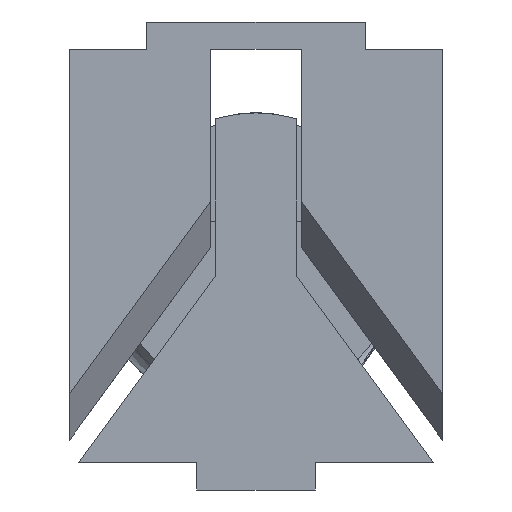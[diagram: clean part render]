
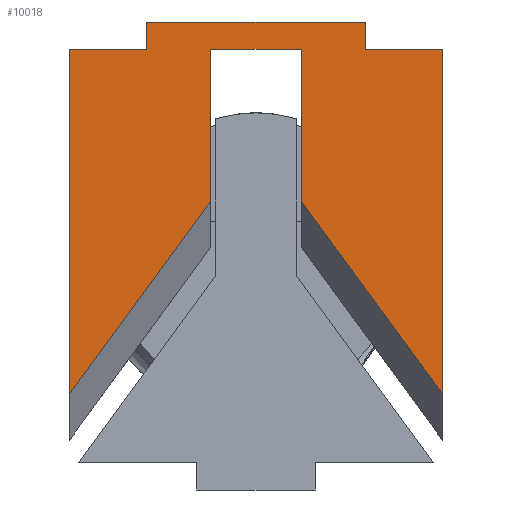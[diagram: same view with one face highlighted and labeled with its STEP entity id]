
A CAD part, front view. The second image highlights one B-rep face of the part: STEP entity #10018.
In plain terms, the highlighted planar face has unit normal (0, -1, 0).
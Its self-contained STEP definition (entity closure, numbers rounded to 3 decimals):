
#302 = VECTOR ( 'NONE', #7998, 1000. ) ;
#310 = ORIENTED_EDGE ( 'NONE', *, *, #9682, .F. ) ;
#428 = VECTOR ( 'NONE', #872, 1000. ) ;
#720 = ORIENTED_EDGE ( 'NONE', *, *, #2847, .T. ) ;
#864 = CARTESIAN_POINT ( 'NONE',  ( -12., 50., 17. ) ) ;
#872 = DIRECTION ( 'NONE',  ( 0., 0., -1. ) ) ;
#1059 = EDGE_CURVE ( 'NONE', #4661, #6381, #4968, .T. ) ;
#1181 = CARTESIAN_POINT ( 'NONE',  ( 20.5, 50., -23.919 ) ) ;
#1329 = ORIENTED_EDGE ( 'NONE', *, *, #1059, .F. ) ;
#1627 = DIRECTION ( 'NONE',  ( 0., 0., 1. ) ) ;
#1660 = CARTESIAN_POINT ( 'NONE',  ( 20.5, 50., 14. ) ) ;
#1767 = EDGE_CURVE ( 'NONE', #5907, #6381, #9399, .T. ) ;
#1841 = VECTOR ( 'NONE', #10079, 1000. ) ;
#1881 = CARTESIAN_POINT ( 'NONE',  ( -12., 50., 17. ) ) ;
#2059 = ORIENTED_EDGE ( 'NONE', *, *, #5242, .T. ) ;
#2090 = VERTEX_POINT ( 'NONE', #6871 ) ;
#2649 = CARTESIAN_POINT ( 'NONE',  ( 0., 50., 14. ) ) ;
#2847 = EDGE_CURVE ( 'NONE', #4973, #5907, #3193, .T. ) ;
#2854 = LINE ( 'NONE', #7149, #2921 ) ;
#2919 = PLANE ( 'NONE',  #5298 ) ;
#2921 = VECTOR ( 'NONE', #5198, 1000. ) ;
#3057 = CARTESIAN_POINT ( 'NONE',  ( 0.665, 50., 3.192 ) ) ;
#3060 = EDGE_CURVE ( 'NONE', #9786, #2090, #2854, .T. ) ;
#3189 = EDGE_CURVE ( 'NONE', #7574, #6319, #8959, .T. ) ;
#3193 = LINE ( 'NONE', #4187, #3800 ) ;
#3325 = CARTESIAN_POINT ( 'NONE',  ( -12., 50., 17. ) ) ;
#3366 = DIRECTION ( 'NONE',  ( 1., 0., 0. ) ) ;
#3448 = EDGE_CURVE ( 'NONE', #3493, #6377, #8599, .T. ) ;
#3468 = LINE ( 'NONE', #864, #9061 ) ;
#3493 = VERTEX_POINT ( 'NONE', #1881 ) ;
#3753 = CARTESIAN_POINT ( 'NONE',  ( -11.822, 50., -12.057 ) ) ;
#3792 = DIRECTION ( 'NONE',  ( 0., 0., 1. ) ) ;
#3800 = VECTOR ( 'NONE', #1627, 1000. ) ;
#4056 = DIRECTION ( 'NONE',  ( 0.59, 0., -0.807 ) ) ;
#4106 = CARTESIAN_POINT ( 'NONE',  ( 5., 50., -2.733 ) ) ;
#4187 = CARTESIAN_POINT ( 'NONE',  ( -5., 50., 0. ) ) ;
#4564 = VERTEX_POINT ( 'NONE', #8479 ) ;
#4588 = CARTESIAN_POINT ( 'NONE',  ( 0., 50., 14. ) ) ;
#4602 = DIRECTION ( 'NONE',  ( 0.59, 0., 0.807 ) ) ;
#4661 = VERTEX_POINT ( 'NONE', #4106 ) ;
#4705 = DIRECTION ( 'NONE',  ( 0., 0., 1. ) ) ;
#4827 = EDGE_CURVE ( 'NONE', #3493, #9786, #3468, .T. ) ;
#4846 = DIRECTION ( 'NONE',  ( 0., 0., -1. ) ) ;
#4892 = LINE ( 'NONE', #3057, #5358 ) ;
#4968 = LINE ( 'NONE', #5805, #8323 ) ;
#4973 = VERTEX_POINT ( 'NONE', #7791 ) ;
#5173 = CARTESIAN_POINT ( 'NONE',  ( -20.5, 50., 14. ) ) ;
#5198 = DIRECTION ( 'NONE',  ( 0., 0., -1. ) ) ;
#5242 = EDGE_CURVE ( 'NONE', #4564, #4973, #9868, .T. ) ;
#5298 = AXIS2_PLACEMENT_3D ( 'NONE', #8280, #6409, #4705 ) ;
#5358 = VECTOR ( 'NONE', #4056, 1000. ) ;
#5729 = CARTESIAN_POINT ( 'NONE',  ( -20.5, 50., 0. ) ) ;
#5780 = VECTOR ( 'NONE', #4846, 1000. ) ;
#5805 = CARTESIAN_POINT ( 'NONE',  ( 5., 50., 0. ) ) ;
#5907 = VERTEX_POINT ( 'NONE', #9472 ) ;
#6319 = VERTEX_POINT ( 'NONE', #1181 ) ;
#6377 = VERTEX_POINT ( 'NONE', #7035 ) ;
#6381 = VERTEX_POINT ( 'NONE', #7280 ) ;
#6409 = DIRECTION ( 'NONE',  ( 0., 1., 0. ) ) ;
#6649 = EDGE_CURVE ( 'NONE', #10498, #4564, #6877, .T. ) ;
#6693 = ORIENTED_EDGE ( 'NONE', *, *, #3060, .F. ) ;
#6871 = CARTESIAN_POINT ( 'NONE',  ( 12., 50., 14. ) ) ;
#6877 = LINE ( 'NONE', #5729, #8265 ) ;
#6915 = ORIENTED_EDGE ( 'NONE', *, *, #3189, .F. ) ;
#7035 = CARTESIAN_POINT ( 'NONE',  ( -12., 50., 14. ) ) ;
#7149 = CARTESIAN_POINT ( 'NONE',  ( 12., 50., 17. ) ) ;
#7280 = CARTESIAN_POINT ( 'NONE',  ( 5., 50., 14. ) ) ;
#7354 = ORIENTED_EDGE ( 'NONE', *, *, #3448, .T. ) ;
#7425 = CARTESIAN_POINT ( 'NONE',  ( 20.5, 50., 0. ) ) ;
#7574 = VERTEX_POINT ( 'NONE', #1660 ) ;
#7791 = CARTESIAN_POINT ( 'NONE',  ( -5., 50., -2.733 ) ) ;
#7901 = EDGE_CURVE ( 'NONE', #4661, #6319, #4892, .T. ) ;
#7962 = EDGE_CURVE ( 'NONE', #10498, #6377, #8637, .T. ) ;
#7998 = DIRECTION ( 'NONE',  ( 1., 0., 0. ) ) ;
#8187 = ORIENTED_EDGE ( 'NONE', *, *, #7901, .T. ) ;
#8228 = FACE_OUTER_BOUND ( 'NONE', #11048, .T. ) ;
#8265 = VECTOR ( 'NONE', #9255, 1000. ) ;
#8280 = CARTESIAN_POINT ( 'NONE',  ( -16., 50., -9. ) ) ;
#8323 = VECTOR ( 'NONE', #3792, 1000. ) ;
#8479 = CARTESIAN_POINT ( 'NONE',  ( -20.5, 50., -23.919 ) ) ;
#8498 = CARTESIAN_POINT ( 'NONE',  ( -12., 50., 14. ) ) ;
#8574 = VECTOR ( 'NONE', #4602, 1000. ) ;
#8599 = LINE ( 'NONE', #3325, #428 ) ;
#8637 = LINE ( 'NONE', #2649, #10555 ) ;
#8784 = ORIENTED_EDGE ( 'NONE', *, *, #6649, .T. ) ;
#8824 = ORIENTED_EDGE ( 'NONE', *, *, #1767, .T. ) ;
#8850 = LINE ( 'NONE', #4588, #302 ) ;
#8959 = LINE ( 'NONE', #7425, #5780 ) ;
#9061 = VECTOR ( 'NONE', #9541, 1000. ) ;
#9165 = ORIENTED_EDGE ( 'NONE', *, *, #4827, .F. ) ;
#9255 = DIRECTION ( 'NONE',  ( 0., 0., -1. ) ) ;
#9281 = ORIENTED_EDGE ( 'NONE', *, *, #7962, .F. ) ;
#9399 = LINE ( 'NONE', #8498, #1841 ) ;
#9472 = CARTESIAN_POINT ( 'NONE',  ( -5., 50., 14. ) ) ;
#9541 = DIRECTION ( 'NONE',  ( 1., 0., 0. ) ) ;
#9682 = EDGE_CURVE ( 'NONE', #2090, #7574, #8850, .T. ) ;
#9786 = VERTEX_POINT ( 'NONE', #10322 ) ;
#9868 = LINE ( 'NONE', #3753, #8574 ) ;
#10018 = ADVANCED_FACE ( 'NONE', ( #8228 ), #2919, .F. ) ;
#10079 = DIRECTION ( 'NONE',  ( 1., 0., 0. ) ) ;
#10322 = CARTESIAN_POINT ( 'NONE',  ( 12., 50., 17. ) ) ;
#10498 = VERTEX_POINT ( 'NONE', #5173 ) ;
#10555 = VECTOR ( 'NONE', #3366, 1000. ) ;
#11048 = EDGE_LOOP ( 'NONE', ( #8784, #2059, #720, #8824, #1329, #8187, #6915, #310, #6693, #9165, #7354, #9281 ) ) ;
